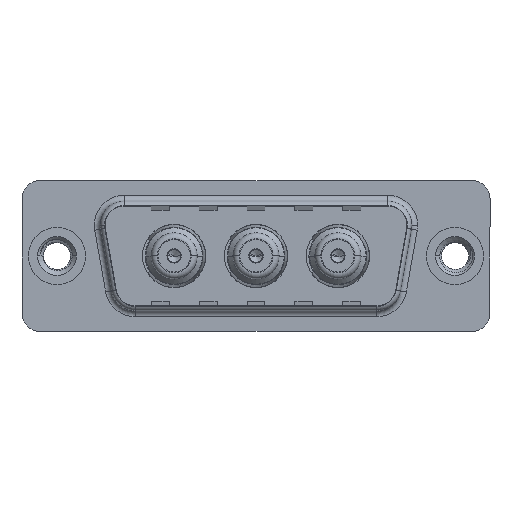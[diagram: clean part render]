
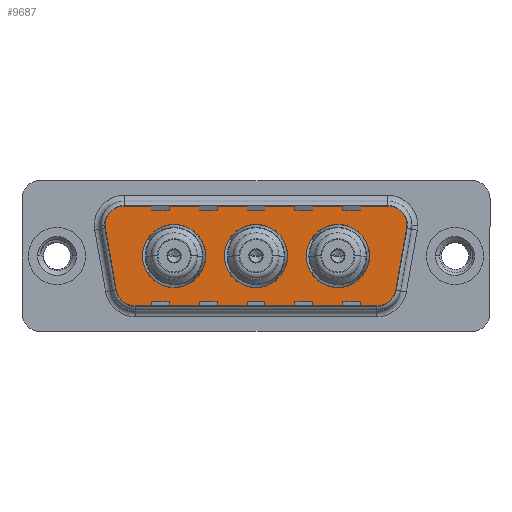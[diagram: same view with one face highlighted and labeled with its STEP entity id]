
A CAD part, top view. The second image highlights one B-rep face of the part: STEP entity #9687.
In plain terms, the highlighted planar face has unit normal (0, 0, 1).
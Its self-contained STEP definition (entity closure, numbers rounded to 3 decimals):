
#110 = FACE_BOUND ( 'NONE', #6045, .T. ) ;
#206 = LINE ( 'NONE', #2176, #7836 ) ;
#325 = AXIS2_PLACEMENT_3D ( 'NONE', #5468, #15174, #6915 ) ;
#380 = LINE ( 'NONE', #11524, #11234 ) ;
#416 = CIRCLE ( 'NONE', #13545, 2.65 ) ;
#763 = DIRECTION ( 'NONE',  ( 0., 0., 1. ) ) ;
#776 = CARTESIAN_POINT ( 'NONE',  ( 12.45, 0., 0. ) ) ;
#859 = LINE ( 'NONE', #15109, #15318 ) ;
#1224 = EDGE_CURVE ( 'NONE', #13664, #8141, #4240, .T. ) ;
#1467 = AXIS2_PLACEMENT_3D ( 'NONE', #15920, #13304, #6222 ) ;
#1513 = AXIS2_PLACEMENT_3D ( 'NONE', #4790, #14517, #6224 ) ;
#1714 = EDGE_CURVE ( 'NONE', #17279, #9340, #2177, .T. ) ;
#1764 = ORIENTED_EDGE ( 'NONE', *, *, #15511, .F. ) ;
#1931 = CARTESIAN_POINT ( 'NONE',  ( 5.411, 4.9, 0. ) ) ;
#2176 = CARTESIAN_POINT ( 'NONE',  ( 29.859, 2.553, 0. ) ) ;
#2177 = CIRCLE ( 'NONE', #7309, 2.65 ) ;
#2203 = CARTESIAN_POINT ( 'NONE',  ( 27.889, 4.9, 0. ) ) ;
#2232 = CARTESIAN_POINT ( 'NONE',  ( 20.85, 0., 0. ) ) ;
#2547 = ORIENTED_EDGE ( 'NONE', *, *, #3277, .T. ) ;
#2630 = CARTESIAN_POINT ( 'NONE',  ( 29.889, 2.9, 0. ) ) ;
#2927 = ORIENTED_EDGE ( 'NONE', *, *, #1714, .F. ) ;
#3019 = AXIS2_PLACEMENT_3D ( 'NONE', #15311, #8507, #18154 ) ;
#3036 = ORIENTED_EDGE ( 'NONE', *, *, #1224, .T. ) ;
#3075 = DIRECTION ( 'NONE',  ( 0.174, -0.985, 0. ) ) ;
#3218 = ORIENTED_EDGE ( 'NONE', *, *, #5187, .T. ) ;
#3277 = EDGE_CURVE ( 'NONE', #14561, #5927, #16695, .T. ) ;
#3457 = CARTESIAN_POINT ( 'NONE',  ( 16.65, 0., 0. ) ) ;
#3613 = ORIENTED_EDGE ( 'NONE', *, *, #6824, .T. ) ;
#3705 = DIRECTION ( 'NONE',  ( 0., 0., 1. ) ) ;
#3828 = DIRECTION ( 'NONE',  ( 1., 0., 0. ) ) ;
#3930 = AXIS2_PLACEMENT_3D ( 'NONE', #9294, #763, #10668 ) ;
#3988 = DIRECTION ( 'NONE',  ( 0., 0., 1. ) ) ;
#4221 = PLANE ( 'NONE',  #3019 ) ;
#4240 = CIRCLE ( 'NONE', #9865, 2. ) ;
#4401 = EDGE_CURVE ( 'NONE', #9340, #17279, #11514, .T. ) ;
#4790 = CARTESIAN_POINT ( 'NONE',  ( 16.65, 0., 0. ) ) ;
#4890 = DIRECTION ( 'NONE',  ( 1., 0., 0. ) ) ;
#4917 = EDGE_CURVE ( 'NONE', #14932, #14608, #206, .T. ) ;
#4947 = EDGE_LOOP ( 'NONE', ( #1764, #14881 ) ) ;
#5187 = EDGE_CURVE ( 'NONE', #8141, #6916, #859, .T. ) ;
#5468 = CARTESIAN_POINT ( 'NONE',  ( 27.889, 2.9, 0. ) ) ;
#5622 = VECTOR ( 'NONE', #14458, 1000. ) ;
#5673 = VERTEX_POINT ( 'NONE', #2232 ) ;
#5745 = CIRCLE ( 'NONE', #7268, 2. ) ;
#5841 = DIRECTION ( 'NONE',  ( 0., 0., 1. ) ) ;
#5859 = CIRCLE ( 'NONE', #3930, 2. ) ;
#5899 = CIRCLE ( 'NONE', #12938, 2. ) ;
#5927 = VERTEX_POINT ( 'NONE', #1931 ) ;
#6045 = EDGE_LOOP ( 'NONE', ( #15472, #12233 ) ) ;
#6110 = CARTESIAN_POINT ( 'NONE',  ( 14., 0., 0. ) ) ;
#6222 = DIRECTION ( 'NONE',  ( 1., 0., 0. ) ) ;
#6224 = DIRECTION ( 'NONE',  ( 1., 0., 0. ) ) ;
#6391 = EDGE_LOOP ( 'NONE', ( #13889, #7706, #11488, #12204, #2547, #3613, #8606, #3036, #3218 ) ) ;
#6478 = CARTESIAN_POINT ( 'NONE',  ( 26.866, -4.9, 0. ) ) ;
#6824 = EDGE_CURVE ( 'NONE', #5927, #14142, #5745, .T. ) ;
#6915 = DIRECTION ( 'NONE',  ( -1., 0., 0. ) ) ;
#6916 = VERTEX_POINT ( 'NONE', #6478 ) ;
#7172 = DIRECTION ( 'NONE',  ( 0., 0., 1. ) ) ;
#7268 = AXIS2_PLACEMENT_3D ( 'NONE', #16750, #3705, #3828 ) ;
#7286 = FACE_OUTER_BOUND ( 'NONE', #6391, .T. ) ;
#7309 = AXIS2_PLACEMENT_3D ( 'NONE', #15599, #15278, #9560 ) ;
#7706 = ORIENTED_EDGE ( 'NONE', *, *, #4917, .T. ) ;
#7788 = CIRCLE ( 'NONE', #1513, 2.65 ) ;
#7836 = VECTOR ( 'NONE', #15695, 1000. ) ;
#8141 = VERTEX_POINT ( 'NONE', #8358 ) ;
#8275 = EDGE_CURVE ( 'NONE', #10214, #11555, #17022, .T. ) ;
#8358 = CARTESIAN_POINT ( 'NONE',  ( 6.434, -4.9, 0. ) ) ;
#8507 = DIRECTION ( 'NONE',  ( 0., 0., 1. ) ) ;
#8537 = CARTESIAN_POINT ( 'NONE',  ( 3.441, 2.553, 0. ) ) ;
#8593 = VERTEX_POINT ( 'NONE', #2630 ) ;
#8606 = ORIENTED_EDGE ( 'NONE', *, *, #16773, .T. ) ;
#8966 = CARTESIAN_POINT ( 'NONE',  ( 4.464, -3.247, 0. ) ) ;
#9294 = CARTESIAN_POINT ( 'NONE',  ( 27.889, 2.9, 0. ) ) ;
#9340 = VERTEX_POINT ( 'NONE', #15752 ) ;
#9560 = DIRECTION ( 'NONE',  ( 1., 0., 0. ) ) ;
#9687 = ADVANCED_FACE ( 'NONE', ( #110, #11406, #10967, #7286 ), #4221, .T. ) ;
#9865 = AXIS2_PLACEMENT_3D ( 'NONE', #15333, #17343, #16399 ) ;
#10214 = VERTEX_POINT ( 'NONE', #10941 ) ;
#10367 = EDGE_CURVE ( 'NONE', #6916, #14932, #5899, .T. ) ;
#10447 = DIRECTION ( 'NONE',  ( 1., 0., 0. ) ) ;
#10668 = DIRECTION ( 'NONE',  ( -1., 0., 0. ) ) ;
#10941 = CARTESIAN_POINT ( 'NONE',  ( 19.3, 0., 0. ) ) ;
#10967 = FACE_BOUND ( 'NONE', #13107, .T. ) ;
#11064 = CIRCLE ( 'NONE', #325, 2. ) ;
#11234 = VECTOR ( 'NONE', #3075, 1000. ) ;
#11406 = FACE_BOUND ( 'NONE', #4947, .T. ) ;
#11488 = ORIENTED_EDGE ( 'NONE', *, *, #12336, .T. ) ;
#11514 = CIRCLE ( 'NONE', #1467, 2.65 ) ;
#11524 = CARTESIAN_POINT ( 'NONE',  ( 3.441, 2.553, 0. ) ) ;
#11555 = VERTEX_POINT ( 'NONE', #6110 ) ;
#11677 = CARTESIAN_POINT ( 'NONE',  ( 26.15, 0., 0. ) ) ;
#12204 = ORIENTED_EDGE ( 'NONE', *, *, #15312, .T. ) ;
#12233 = ORIENTED_EDGE ( 'NONE', *, *, #17102, .F. ) ;
#12336 = EDGE_CURVE ( 'NONE', #14608, #8593, #5859, .T. ) ;
#12372 = CARTESIAN_POINT ( 'NONE',  ( 23.5, 0., 0. ) ) ;
#12542 = EDGE_CURVE ( 'NONE', #5673, #17870, #13905, .T. ) ;
#12664 = AXIS2_PLACEMENT_3D ( 'NONE', #3457, #13265, #4890 ) ;
#12938 = AXIS2_PLACEMENT_3D ( 'NONE', #15412, #7172, #16826 ) ;
#13107 = EDGE_LOOP ( 'NONE', ( #2927, #16975 ) ) ;
#13265 = DIRECTION ( 'NONE',  ( 0., 0., 1. ) ) ;
#13285 = AXIS2_PLACEMENT_3D ( 'NONE', #12372, #3988, #13740 ) ;
#13304 = DIRECTION ( 'NONE',  ( 0., 0., 1. ) ) ;
#13510 = CARTESIAN_POINT ( 'NONE',  ( 29.859, 2.553, 0. ) ) ;
#13545 = AXIS2_PLACEMENT_3D ( 'NONE', #14164, #5841, #15526 ) ;
#13664 = VERTEX_POINT ( 'NONE', #8966 ) ;
#13740 = DIRECTION ( 'NONE',  ( 1., 0., 0. ) ) ;
#13889 = ORIENTED_EDGE ( 'NONE', *, *, #10367, .T. ) ;
#13905 = CIRCLE ( 'NONE', #13285, 2.65 ) ;
#14142 = VERTEX_POINT ( 'NONE', #8537 ) ;
#14164 = CARTESIAN_POINT ( 'NONE',  ( 23.5, 0., 0. ) ) ;
#14458 = DIRECTION ( 'NONE',  ( -1., 0., 0. ) ) ;
#14517 = DIRECTION ( 'NONE',  ( 0., 0., 1. ) ) ;
#14526 = CARTESIAN_POINT ( 'NONE',  ( 28.836, -3.247, 0. ) ) ;
#14561 = VERTEX_POINT ( 'NONE', #2203 ) ;
#14608 = VERTEX_POINT ( 'NONE', #13510 ) ;
#14881 = ORIENTED_EDGE ( 'NONE', *, *, #12542, .F. ) ;
#14932 = VERTEX_POINT ( 'NONE', #14526 ) ;
#15109 = CARTESIAN_POINT ( 'NONE',  ( 6.434, -4.9, 0. ) ) ;
#15174 = DIRECTION ( 'NONE',  ( 0., 0., 1. ) ) ;
#15278 = DIRECTION ( 'NONE',  ( 0., 0., 1. ) ) ;
#15311 = CARTESIAN_POINT ( 'NONE',  ( 26.866, -2.9, 0. ) ) ;
#15312 = EDGE_CURVE ( 'NONE', #8593, #14561, #11064, .T. ) ;
#15318 = VECTOR ( 'NONE', #10447, 1000. ) ;
#15333 = CARTESIAN_POINT ( 'NONE',  ( 6.434, -2.9, 0. ) ) ;
#15412 = CARTESIAN_POINT ( 'NONE',  ( 26.866, -2.9, 0. ) ) ;
#15472 = ORIENTED_EDGE ( 'NONE', *, *, #8275, .F. ) ;
#15511 = EDGE_CURVE ( 'NONE', #17870, #5673, #416, .T. ) ;
#15526 = DIRECTION ( 'NONE',  ( 1., 0., 0. ) ) ;
#15599 = CARTESIAN_POINT ( 'NONE',  ( 9.8, 0., 0. ) ) ;
#15695 = DIRECTION ( 'NONE',  ( 0.174, 0.985, 0. ) ) ;
#15752 = CARTESIAN_POINT ( 'NONE',  ( 7.15, 0., 0. ) ) ;
#15920 = CARTESIAN_POINT ( 'NONE',  ( 9.8, 0., 0. ) ) ;
#16399 = DIRECTION ( 'NONE',  ( -1., 0., 0. ) ) ;
#16695 = LINE ( 'NONE', #17854, #5622 ) ;
#16750 = CARTESIAN_POINT ( 'NONE',  ( 5.411, 2.9, 0. ) ) ;
#16773 = EDGE_CURVE ( 'NONE', #14142, #13664, #380, .T. ) ;
#16826 = DIRECTION ( 'NONE',  ( 1., 0., 0. ) ) ;
#16975 = ORIENTED_EDGE ( 'NONE', *, *, #4401, .F. ) ;
#17022 = CIRCLE ( 'NONE', #12664, 2.65 ) ;
#17102 = EDGE_CURVE ( 'NONE', #11555, #10214, #7788, .T. ) ;
#17279 = VERTEX_POINT ( 'NONE', #776 ) ;
#17343 = DIRECTION ( 'NONE',  ( 0., 0., 1. ) ) ;
#17854 = CARTESIAN_POINT ( 'NONE',  ( 5.411, 4.9, 0. ) ) ;
#17870 = VERTEX_POINT ( 'NONE', #11677 ) ;
#18154 = DIRECTION ( 'NONE',  ( 1., 0., 0. ) ) ;
